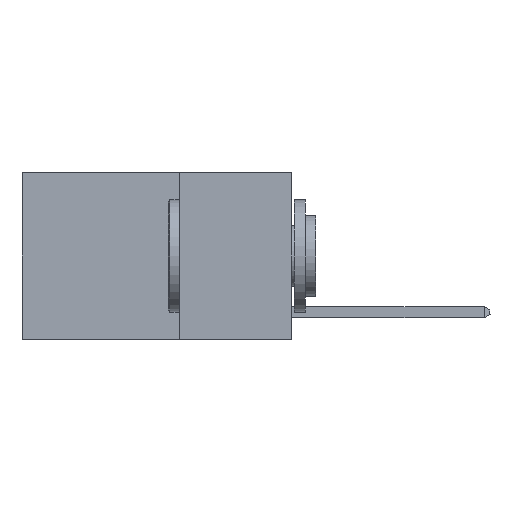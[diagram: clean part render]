
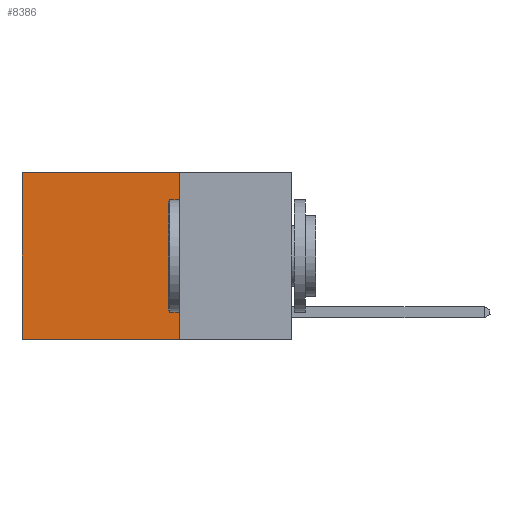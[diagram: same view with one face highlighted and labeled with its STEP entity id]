
A CAD part, left-side view. The second image highlights one B-rep face of the part: STEP entity #8386.
In plain terms, the highlighted planar face has unit normal (-1, 0, 0).
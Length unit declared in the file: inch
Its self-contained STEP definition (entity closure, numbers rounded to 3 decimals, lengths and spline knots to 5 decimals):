
#78 = AXIS2_PLACEMENT_3D ( 'NONE', #10892, #1173, #5524 ) ;
#230 = EDGE_CURVE ( 'NONE', #10372, #7729, #4485, .T. ) ;
#280 = CARTESIAN_POINT ( 'NONE',  ( 0.2625, 0.6, -0.37 ) ) ;
#1173 = DIRECTION ( 'NONE',  ( 1., 0., 0. ) ) ;
#2266 = EDGE_CURVE ( 'NONE', #8571, #7928, #8400, .T. ) ;
#2945 = CARTESIAN_POINT ( 'NONE',  ( 0.2625, 0.25, 0. ) ) ;
#3242 = FACE_OUTER_BOUND ( 'NONE', #5414, .T. ) ;
#4008 = ORIENTED_EDGE ( 'NONE', *, *, #8552, .F. ) ;
#4306 = CARTESIAN_POINT ( 'NONE',  ( 0.2625, 0.25, 0. ) ) ;
#4485 = LINE ( 'NONE', #4555, #12693 ) ;
#4555 = CARTESIAN_POINT ( 'NONE',  ( 0.2625, 0.25, -0.37 ) ) ;
#5146 = ORIENTED_EDGE ( 'NONE', *, *, #230, .F. ) ;
#5414 = EDGE_LOOP ( 'NONE', ( #7631, #5146, #4008, #7066 ) ) ;
#5524 = DIRECTION ( 'NONE',  ( 0., 0., -1. ) ) ;
#5632 = CARTESIAN_POINT ( 'NONE',  ( 0.2625, 0.25, -0.37 ) ) ;
#5999 = VECTOR ( 'NONE', #8394, 39.37008 ) ;
#6076 = VECTOR ( 'NONE', #10676, 39.37008 ) ;
#7066 = ORIENTED_EDGE ( 'NONE', *, *, #2266, .T. ) ;
#7417 = CARTESIAN_POINT ( 'NONE',  ( 0.2625, 0.6, 0. ) ) ;
#7626 = PLANE ( 'NONE',  #78 ) ;
#7631 = ORIENTED_EDGE ( 'NONE', *, *, #8248, .T. ) ;
#7729 = VERTEX_POINT ( 'NONE', #280 ) ;
#7928 = VERTEX_POINT ( 'NONE', #12070 ) ;
#8248 = EDGE_CURVE ( 'NONE', #7928, #7729, #12819, .T. ) ;
#8386 = ADVANCED_FACE ( 'NONE', ( #3242 ), #7626, .F. ) ;
#8394 = DIRECTION ( 'NONE',  ( 0., 0., -1. ) ) ;
#8400 = LINE ( 'NONE', #4306, #6076 ) ;
#8552 = EDGE_CURVE ( 'NONE', #8571, #10372, #13643, .T. ) ;
#8571 = VERTEX_POINT ( 'NONE', #2945 ) ;
#8869 = DIRECTION ( 'NONE',  ( 0., 1., 0. ) ) ;
#10372 = VERTEX_POINT ( 'NONE', #5632 ) ;
#10676 = DIRECTION ( 'NONE',  ( 0., 1., 0. ) ) ;
#10892 = CARTESIAN_POINT ( 'NONE',  ( 0.2625, 0.25, 0. ) ) ;
#11742 = DIRECTION ( 'NONE',  ( 0., 0., -1. ) ) ;
#12070 = CARTESIAN_POINT ( 'NONE',  ( 0.2625, 0.6, 0. ) ) ;
#12562 = VECTOR ( 'NONE', #11742, 39.37008 ) ;
#12662 = CARTESIAN_POINT ( 'NONE',  ( 0.2625, 0.25, 0. ) ) ;
#12693 = VECTOR ( 'NONE', #8869, 39.37008 ) ;
#12819 = LINE ( 'NONE', #7417, #12562 ) ;
#13643 = LINE ( 'NONE', #12662, #5999 ) ;
